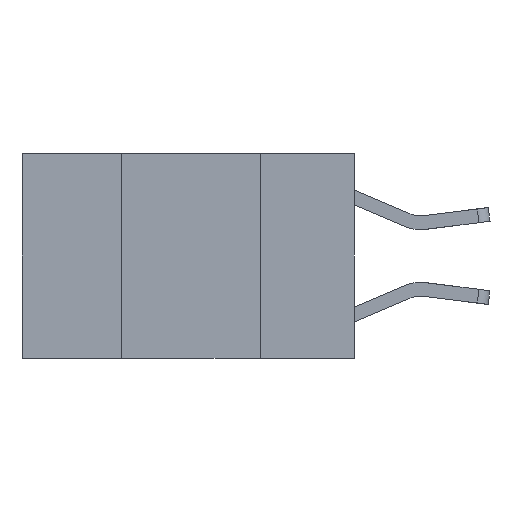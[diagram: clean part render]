
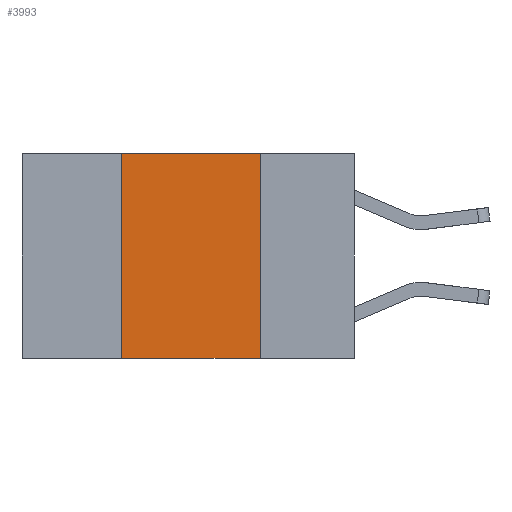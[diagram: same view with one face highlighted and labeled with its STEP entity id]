
A CAD part, left-side view. The second image highlights one B-rep face of the part: STEP entity #3993.
In plain terms, the highlighted planar face has unit normal (-1, 0, 0).
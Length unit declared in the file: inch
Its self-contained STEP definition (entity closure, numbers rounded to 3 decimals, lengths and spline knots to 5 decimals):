
#36 = EDGE_CURVE ( 'NONE', #2642, #6518, #5737, .T. ) ;
#604 = DIRECTION ( 'NONE',  ( 0., 0., 1. ) ) ;
#910 = ORIENTED_EDGE ( 'NONE', *, *, #1952, .F. ) ;
#991 = LINE ( 'NONE', #8615, #5919 ) ;
#1107 = CARTESIAN_POINT ( 'NONE',  ( 0., 0.17, 0. ) ) ;
#1375 = VERTEX_POINT ( 'NONE', #7634 ) ;
#1471 = CARTESIAN_POINT ( 'NONE',  ( 0., 0.6, -0.37 ) ) ;
#1890 = DIRECTION ( 'NONE',  ( 0., -1., 0. ) ) ;
#1952 = EDGE_CURVE ( 'NONE', #6518, #1375, #991, .T. ) ;
#2019 = LINE ( 'NONE', #7495, #7568 ) ;
#2541 = EDGE_CURVE ( 'NONE', #7173, #2642, #2019, .T. ) ;
#2642 = VERTEX_POINT ( 'NONE', #3822 ) ;
#3142 = VECTOR ( 'NONE', #1890, 39.37008 ) ;
#3185 = ORIENTED_EDGE ( 'NONE', *, *, #7699, .T. ) ;
#3822 = CARTESIAN_POINT ( 'NONE',  ( 0., 0.42, 0. ) ) ;
#3993 = ADVANCED_FACE ( 'NONE', ( #4535 ), #7649, .F. ) ;
#4535 = FACE_OUTER_BOUND ( 'NONE', #9202, .T. ) ;
#5189 = VECTOR ( 'NONE', #5469, 39.37008 ) ;
#5469 = DIRECTION ( 'NONE',  ( 0., -1., 0. ) ) ;
#5630 = DIRECTION ( 'NONE',  ( 0., 0., -1. ) ) ;
#5737 = LINE ( 'NONE', #8827, #3142 ) ;
#5919 = VECTOR ( 'NONE', #5630, 39.37008 ) ;
#6518 = VERTEX_POINT ( 'NONE', #1107 ) ;
#6786 = DIRECTION ( 'NONE',  ( 1., 0., 0. ) ) ;
#7173 = VERTEX_POINT ( 'NONE', #7762 ) ;
#7495 = CARTESIAN_POINT ( 'NONE',  ( 0., 0.42, 0. ) ) ;
#7554 = CARTESIAN_POINT ( 'NONE',  ( 0., 0.6, 0. ) ) ;
#7568 = VECTOR ( 'NONE', #604, 39.37008 ) ;
#7634 = CARTESIAN_POINT ( 'NONE',  ( 0., 0.17, -0.37 ) ) ;
#7649 = PLANE ( 'NONE',  #8234 ) ;
#7699 = EDGE_CURVE ( 'NONE', #7173, #1375, #8400, .T. ) ;
#7762 = CARTESIAN_POINT ( 'NONE',  ( 0., 0.42, -0.37 ) ) ;
#8035 = ORIENTED_EDGE ( 'NONE', *, *, #36, .F. ) ;
#8234 = AXIS2_PLACEMENT_3D ( 'NONE', #7554, #6786, #9879 ) ;
#8400 = LINE ( 'NONE', #1471, #5189 ) ;
#8615 = CARTESIAN_POINT ( 'NONE',  ( 0., 0.17, 0. ) ) ;
#8827 = CARTESIAN_POINT ( 'NONE',  ( 0., 0.6, 0. ) ) ;
#9202 = EDGE_LOOP ( 'NONE', ( #910, #8035, #9936, #3185 ) ) ;
#9879 = DIRECTION ( 'NONE',  ( 0., 0., -1. ) ) ;
#9936 = ORIENTED_EDGE ( 'NONE', *, *, #2541, .F. ) ;
